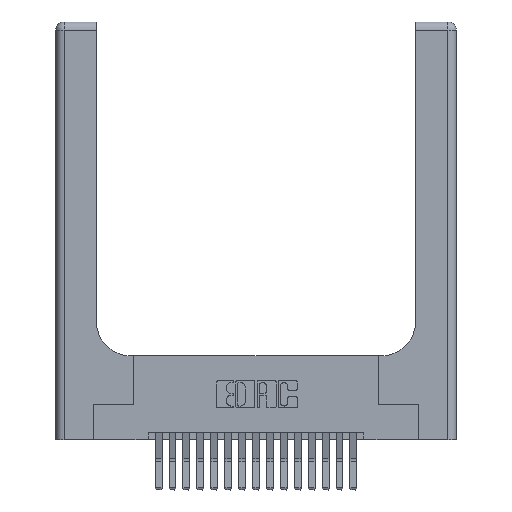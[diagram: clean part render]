
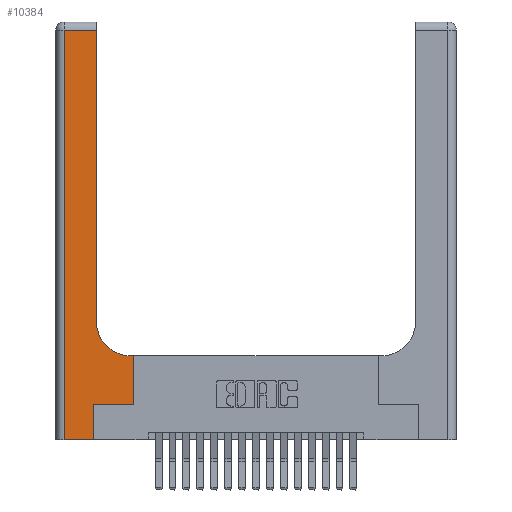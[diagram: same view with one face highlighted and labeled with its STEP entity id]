
A CAD part, top view. The second image highlights one B-rep face of the part: STEP entity #10384.
In plain terms, the highlighted planar face has unit normal (0, 0, 1).
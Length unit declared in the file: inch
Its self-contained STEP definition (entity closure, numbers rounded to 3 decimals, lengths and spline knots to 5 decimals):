
#427 = EDGE_CURVE ( 'NONE', #20462, #15009, #8012, .T. ) ;
#650 = DIRECTION ( 'NONE',  ( 1., 0., 0. ) ) ;
#946 = LINE ( 'NONE', #1872, #13345 ) ;
#1157 = ORIENTED_EDGE ( 'NONE', *, *, #18996, .T. ) ;
#1511 = ORIENTED_EDGE ( 'NONE', *, *, #16570, .T. ) ;
#1833 = CARTESIAN_POINT ( 'NONE',  ( 0.2915, 0.85, 0.37 ) ) ;
#1872 = CARTESIAN_POINT ( 'NONE',  ( 0.5585, 0.25, 0.37 ) ) ;
#1970 = ORIENTED_EDGE ( 'NONE', *, *, #19841, .T. ) ;
#2015 = AXIS2_PLACEMENT_3D ( 'NONE', #13149, #6840, #17820 ) ;
#2336 = CARTESIAN_POINT ( 'NONE',  ( 0.5585, 0.6, 0.37 ) ) ;
#2354 = ORIENTED_EDGE ( 'NONE', *, *, #11860, .T. ) ;
#2389 = CARTESIAN_POINT ( 'NONE',  ( 0.5415, 0.6, 0.37 ) ) ;
#3563 = DIRECTION ( 'NONE',  ( 0., 1., 0. ) ) ;
#3938 = AXIS2_PLACEMENT_3D ( 'NONE', #19772, #10410, #650 ) ;
#3968 = CARTESIAN_POINT ( 'NONE',  ( 0.269, 0.25, 0.37 ) ) ;
#4123 = VECTOR ( 'NONE', #18997, 39.37008 ) ;
#4186 = FACE_OUTER_BOUND ( 'NONE', #13571, .T. ) ;
#4603 = CARTESIAN_POINT ( 'NONE',  ( 0.06, 2.94, 0.37 ) ) ;
#4873 = DIRECTION ( 'NONE',  ( 0., 1., 0. ) ) ;
#5049 = ORIENTED_EDGE ( 'NONE', *, *, #9321, .T. ) ;
#5198 = LINE ( 'NONE', #3968, #17760 ) ;
#5276 = CARTESIAN_POINT ( 'NONE',  ( 0.2915, 0.6, 0.37 ) ) ;
#5455 = CARTESIAN_POINT ( 'NONE',  ( 0., 0., 0.37 ) ) ;
#5687 = CARTESIAN_POINT ( 'NONE',  ( 0., 2.94, 0.37 ) ) ;
#6119 = VERTEX_POINT ( 'NONE', #14676 ) ;
#6739 = VERTEX_POINT ( 'NONE', #2389 ) ;
#6840 = DIRECTION ( 'NONE',  ( 0., 0., -1. ) ) ;
#6884 = DIRECTION ( 'NONE',  ( -1., 0., 0. ) ) ;
#6934 = VECTOR ( 'NONE', #6884, 39.37008 ) ;
#7771 = VECTOR ( 'NONE', #8672, 39.37008 ) ;
#8012 = LINE ( 'NONE', #5687, #19021 ) ;
#8509 = VERTEX_POINT ( 'NONE', #1833 ) ;
#8672 = DIRECTION ( 'NONE',  ( 1., 0., 0. ) ) ;
#9054 = DIRECTION ( 'NONE',  ( -1., 0., 0. ) ) ;
#9108 = DIRECTION ( 'NONE',  ( 0., 1., 0. ) ) ;
#9138 = ORIENTED_EDGE ( 'NONE', *, *, #14708, .T. ) ;
#9258 = CARTESIAN_POINT ( 'NONE',  ( 0.06, 0., 0.37 ) ) ;
#9321 = EDGE_CURVE ( 'NONE', #8509, #20462, #17331, .T. ) ;
#9521 = VECTOR ( 'NONE', #9108, 39.37008 ) ;
#10384 = ADVANCED_FACE ( 'NONE', ( #4186 ), #16262, .F. ) ;
#10410 = DIRECTION ( 'NONE',  ( 0., 0., -1. ) ) ;
#10914 = EDGE_CURVE ( 'NONE', #18470, #6739, #15315, .T. ) ;
#11388 = CARTESIAN_POINT ( 'NONE',  ( 0.2915, 2.94, 0.37 ) ) ;
#11860 = EDGE_CURVE ( 'NONE', #15009, #20305, #16253, .T. ) ;
#11985 = EDGE_CURVE ( 'NONE', #16398, #18470, #946, .T. ) ;
#12849 = CARTESIAN_POINT ( 'NONE',  ( 0.06, 3., 0.37 ) ) ;
#13149 = CARTESIAN_POINT ( 'NONE',  ( 0., 3., 0.37 ) ) ;
#13345 = VECTOR ( 'NONE', #3563, 39.37008 ) ;
#13571 = EDGE_LOOP ( 'NONE', ( #5049, #15839, #2354, #9138, #1970, #1157, #15858, #14265, #1511 ) ) ;
#14265 = ORIENTED_EDGE ( 'NONE', *, *, #10914, .T. ) ;
#14676 = CARTESIAN_POINT ( 'NONE',  ( 0.269, 0., 0.37 ) ) ;
#14708 = EDGE_CURVE ( 'NONE', #20305, #6119, #16143, .T. ) ;
#14918 = CARTESIAN_POINT ( 'NONE',  ( 0.269, 0.25, 0.37 ) ) ;
#15009 = VERTEX_POINT ( 'NONE', #4603 ) ;
#15050 = DIRECTION ( 'NONE',  ( 1., 0., 0. ) ) ;
#15084 = CIRCLE ( 'NONE', #3938, 0.25 ) ;
#15315 = LINE ( 'NONE', #5276, #6934 ) ;
#15839 = ORIENTED_EDGE ( 'NONE', *, *, #427, .T. ) ;
#15858 = ORIENTED_EDGE ( 'NONE', *, *, #11985, .T. ) ;
#16024 = VECTOR ( 'NONE', #4873, 39.37008 ) ;
#16143 = LINE ( 'NONE', #5455, #7771 ) ;
#16253 = LINE ( 'NONE', #12849, #4123 ) ;
#16262 = PLANE ( 'NONE',  #2015 ) ;
#16398 = VERTEX_POINT ( 'NONE', #17782 ) ;
#16570 = EDGE_CURVE ( 'NONE', #6739, #8509, #15084, .T. ) ;
#16894 = CARTESIAN_POINT ( 'NONE',  ( 0.2915, 3., 0.37 ) ) ;
#17249 = VERTEX_POINT ( 'NONE', #14918 ) ;
#17331 = LINE ( 'NONE', #16894, #9521 ) ;
#17397 = CARTESIAN_POINT ( 'NONE',  ( 0.269, 0., 0.37 ) ) ;
#17760 = VECTOR ( 'NONE', #15050, 39.37008 ) ;
#17782 = CARTESIAN_POINT ( 'NONE',  ( 0.5585, 0.25, 0.37 ) ) ;
#17820 = DIRECTION ( 'NONE',  ( -1., 0., 0. ) ) ;
#18470 = VERTEX_POINT ( 'NONE', #2336 ) ;
#18996 = EDGE_CURVE ( 'NONE', #17249, #16398, #5198, .T. ) ;
#18997 = DIRECTION ( 'NONE',  ( 0., -1., 0. ) ) ;
#19021 = VECTOR ( 'NONE', #9054, 39.37008 ) ;
#19689 = LINE ( 'NONE', #17397, #16024 ) ;
#19772 = CARTESIAN_POINT ( 'NONE',  ( 0.5415, 0.85, 0.37 ) ) ;
#19841 = EDGE_CURVE ( 'NONE', #6119, #17249, #19689, .T. ) ;
#20305 = VERTEX_POINT ( 'NONE', #9258 ) ;
#20462 = VERTEX_POINT ( 'NONE', #11388 ) ;
